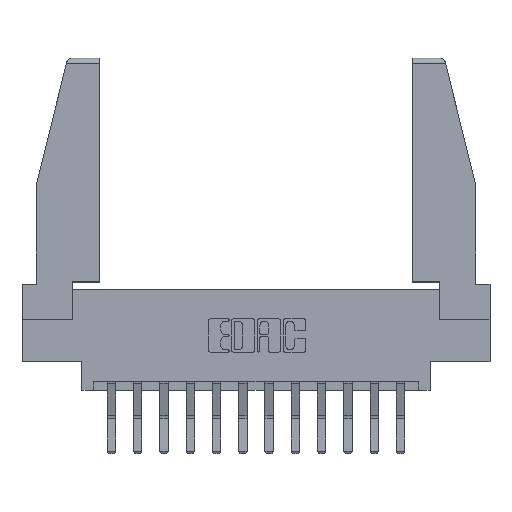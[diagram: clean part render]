
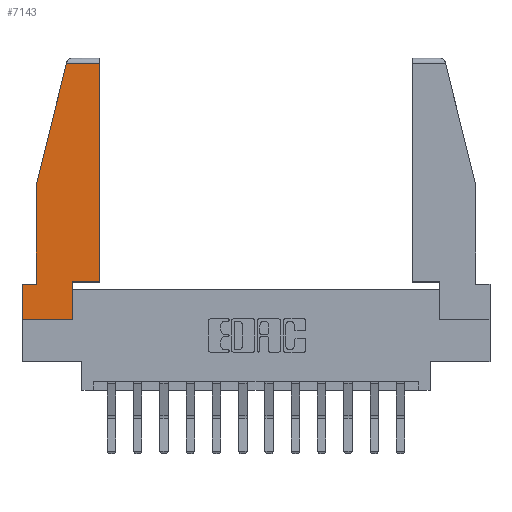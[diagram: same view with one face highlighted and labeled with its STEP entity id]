
A CAD part, top view. The second image highlights one B-rep face of the part: STEP entity #7143.
In plain terms, the highlighted planar face has unit normal (0, 0, 1).
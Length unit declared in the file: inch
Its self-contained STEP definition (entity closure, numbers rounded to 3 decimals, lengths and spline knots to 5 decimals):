
#419 = VERTEX_POINT ( 'NONE', #3606 ) ;
#735 = VECTOR ( 'NONE', #2374, 39.37008 ) ;
#849 = VERTEX_POINT ( 'NONE', #13824 ) ;
#1309 = ORIENTED_EDGE ( 'NONE', *, *, #10737, .T. ) ;
#1400 = FACE_OUTER_BOUND ( 'NONE', #4951, .T. ) ;
#1496 = DIRECTION ( 'NONE',  ( 0., -1., 0. ) ) ;
#1586 = ORIENTED_EDGE ( 'NONE', *, *, #5918, .T. ) ;
#2023 = VECTOR ( 'NONE', #7428, 39.37008 ) ;
#2229 = CARTESIAN_POINT ( 'NONE',  ( 0., 0., 0. ) ) ;
#2367 = EDGE_CURVE ( 'NONE', #419, #13725, #7572, .T. ) ;
#2374 = DIRECTION ( 'NONE',  ( 1., 0., 0. ) ) ;
#2523 = EDGE_CURVE ( 'NONE', #5554, #14835, #8326, .T. ) ;
#2571 = CARTESIAN_POINT ( 'NONE',  ( 0.297, 0., 0. ) ) ;
#2669 = VECTOR ( 'NONE', #10981, 39.37008 ) ;
#2706 = PLANE ( 'NONE',  #10455 ) ;
#2853 = CARTESIAN_POINT ( 'NONE',  ( 0.297, 0.223, 0. ) ) ;
#2932 = VECTOR ( 'NONE', #15061, 39.37008 ) ;
#3418 = VERTEX_POINT ( 'NONE', #3679 ) ;
#3572 = LINE ( 'NONE', #2571, #4699 ) ;
#3574 = VERTEX_POINT ( 'NONE', #9931 ) ;
#3579 = CARTESIAN_POINT ( 'NONE',  ( 0.271, 1.55, 0. ) ) ;
#3606 = CARTESIAN_POINT ( 'NONE',  ( 0.086, 0.8, 0. ) ) ;
#3650 = VECTOR ( 'NONE', #10736, 39.37008 ) ;
#3655 = CARTESIAN_POINT ( 'NONE',  ( 0., 0.21, 0. ) ) ;
#3679 = CARTESIAN_POINT ( 'NONE',  ( 0.2636, 1.52, 0. ) ) ;
#3903 = CARTESIAN_POINT ( 'NONE',  ( 0., 0., 0. ) ) ;
#4168 = CARTESIAN_POINT ( 'NONE',  ( 0., 1.52, 0. ) ) ;
#4693 = CARTESIAN_POINT ( 'NONE',  ( 0.297, 0.223, 0. ) ) ;
#4699 = VECTOR ( 'NONE', #9977, 39.37008 ) ;
#4894 = EDGE_CURVE ( 'NONE', #849, #9178, #7697, .T. ) ;
#4923 = LINE ( 'NONE', #4693, #735 ) ;
#4928 = CARTESIAN_POINT ( 'NONE',  ( 0., 0.21, 0. ) ) ;
#4951 = EDGE_LOOP ( 'NONE', ( #8343, #1309, #13628, #7963, #12634, #13346, #1586, #7984, #7659 ) ) ;
#5327 = VECTOR ( 'NONE', #14821, 39.37008 ) ;
#5508 = LINE ( 'NONE', #3579, #2669 ) ;
#5554 = VERTEX_POINT ( 'NONE', #3655 ) ;
#5618 = VECTOR ( 'NONE', #1496, 39.37008 ) ;
#5918 = EDGE_CURVE ( 'NONE', #14835, #3574, #14478, .T. ) ;
#6506 = VERTEX_POINT ( 'NONE', #2853 ) ;
#7143 = ADVANCED_FACE ( 'NONE', ( #1400 ), #2706, .T. ) ;
#7428 = DIRECTION ( 'NONE',  ( 1., 0., 0. ) ) ;
#7572 = LINE ( 'NONE', #15128, #10273 ) ;
#7617 = CARTESIAN_POINT ( 'NONE',  ( 0., 0.21, 0. ) ) ;
#7632 = DIRECTION ( 'NONE',  ( 0., -1., 0. ) ) ;
#7659 = ORIENTED_EDGE ( 'NONE', *, *, #12765, .T. ) ;
#7697 = LINE ( 'NONE', #9525, #3650 ) ;
#7963 = ORIENTED_EDGE ( 'NONE', *, *, #2367, .T. ) ;
#7984 = ORIENTED_EDGE ( 'NONE', *, *, #8476, .T. ) ;
#8326 = LINE ( 'NONE', #7617, #5618 ) ;
#8343 = ORIENTED_EDGE ( 'NONE', *, *, #4894, .T. ) ;
#8476 = EDGE_CURVE ( 'NONE', #3574, #6506, #3572, .T. ) ;
#8484 = CARTESIAN_POINT ( 'NONE',  ( 0.086, 0.21, 0. ) ) ;
#8741 = DIRECTION ( 'NONE',  ( 0., 0., 1. ) ) ;
#9178 = VERTEX_POINT ( 'NONE', #14246 ) ;
#9525 = CARTESIAN_POINT ( 'NONE',  ( 0.461, 0.223, 0. ) ) ;
#9786 = LINE ( 'NONE', #4928, #5327 ) ;
#9841 = LINE ( 'NONE', #4168, #2932 ) ;
#9931 = CARTESIAN_POINT ( 'NONE',  ( 0.297, 0., 0. ) ) ;
#9977 = DIRECTION ( 'NONE',  ( 0., 1., 0. ) ) ;
#10273 = VECTOR ( 'NONE', #7632, 39.37008 ) ;
#10455 = AXIS2_PLACEMENT_3D ( 'NONE', #3903, #8741, #14893 ) ;
#10736 = DIRECTION ( 'NONE',  ( 0., 1., 0. ) ) ;
#10737 = EDGE_CURVE ( 'NONE', #9178, #3418, #9841, .T. ) ;
#10981 = DIRECTION ( 'NONE',  ( -0.239, -0.971, 0. ) ) ;
#12493 = EDGE_CURVE ( 'NONE', #13725, #5554, #9786, .T. ) ;
#12634 = ORIENTED_EDGE ( 'NONE', *, *, #12493, .T. ) ;
#12765 = EDGE_CURVE ( 'NONE', #6506, #849, #4923, .T. ) ;
#13346 = ORIENTED_EDGE ( 'NONE', *, *, #2523, .T. ) ;
#13628 = ORIENTED_EDGE ( 'NONE', *, *, #13646, .T. ) ;
#13646 = EDGE_CURVE ( 'NONE', #3418, #419, #5508, .T. ) ;
#13725 = VERTEX_POINT ( 'NONE', #8484 ) ;
#13824 = CARTESIAN_POINT ( 'NONE',  ( 0.461, 0.223, 0. ) ) ;
#14220 = CARTESIAN_POINT ( 'NONE',  ( 0., 0., 0. ) ) ;
#14246 = CARTESIAN_POINT ( 'NONE',  ( 0.461, 1.52, 0. ) ) ;
#14478 = LINE ( 'NONE', #2229, #2023 ) ;
#14821 = DIRECTION ( 'NONE',  ( -1., 0., 0. ) ) ;
#14835 = VERTEX_POINT ( 'NONE', #14220 ) ;
#14893 = DIRECTION ( 'NONE',  ( 1., 0., 0. ) ) ;
#15061 = DIRECTION ( 'NONE',  ( -1., 0., 0. ) ) ;
#15128 = CARTESIAN_POINT ( 'NONE',  ( 0.086, 0.8, 0. ) ) ;
